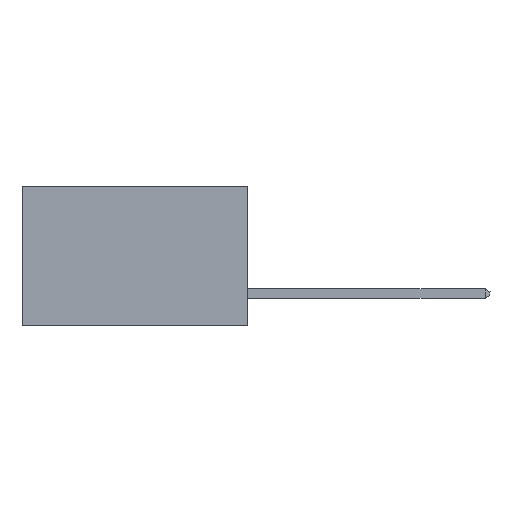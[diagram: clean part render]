
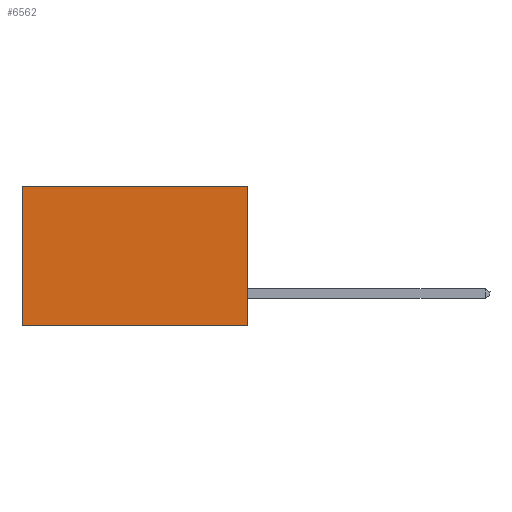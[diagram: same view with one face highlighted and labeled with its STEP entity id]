
A CAD part, left-side view. The second image highlights one B-rep face of the part: STEP entity #6562.
In plain terms, the highlighted planar face has unit normal (-1, 0, 0).
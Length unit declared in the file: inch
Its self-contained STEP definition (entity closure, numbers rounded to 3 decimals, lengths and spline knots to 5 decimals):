
#24 = VERTEX_POINT ( 'NONE', #7957 ) ;
#61 = EDGE_CURVE ( 'NONE', #7415, #7233, #4012, .T. ) ;
#595 = CARTESIAN_POINT ( 'NONE',  ( 0.2615, 0., -0.37 ) ) ;
#626 = CARTESIAN_POINT ( 'NONE',  ( 0.2615, 0., -0.37 ) ) ;
#1001 = DIRECTION ( 'NONE',  ( 1., 0., 0. ) ) ;
#1233 = LINE ( 'NONE', #626, #4310 ) ;
#1252 = DIRECTION ( 'NONE',  ( 0., 0., -1. ) ) ;
#1678 = VERTEX_POINT ( 'NONE', #8600 ) ;
#1913 = EDGE_CURVE ( 'NONE', #1678, #7233, #5636, .T. ) ;
#2053 = DIRECTION ( 'NONE',  ( 0., 0., -1. ) ) ;
#2058 = ORIENTED_EDGE ( 'NONE', *, *, #7206, .T. ) ;
#2691 = VECTOR ( 'NONE', #4969, 39.37008 ) ;
#2714 = EDGE_LOOP ( 'NONE', ( #5445, #8062, #8939, #2058 ) ) ;
#3374 = CARTESIAN_POINT ( 'NONE',  ( 0.2615, 0.6, -0.37 ) ) ;
#3808 = DIRECTION ( 'NONE',  ( 0., 0., -1. ) ) ;
#3899 = PLANE ( 'NONE',  #4866 ) ;
#4012 = LINE ( 'NONE', #3374, #8035 ) ;
#4310 = VECTOR ( 'NONE', #2053, 39.37008 ) ;
#4866 = AXIS2_PLACEMENT_3D ( 'NONE', #6674, #1001, #3808 ) ;
#4880 = CARTESIAN_POINT ( 'NONE',  ( 0.2615, 0., 0. ) ) ;
#4969 = DIRECTION ( 'NONE',  ( 0., 1., 0. ) ) ;
#5445 = ORIENTED_EDGE ( 'NONE', *, *, #61, .T. ) ;
#5636 = LINE ( 'NONE', #595, #6401 ) ;
#6177 = DIRECTION ( 'NONE',  ( 0., 1., 0. ) ) ;
#6244 = LINE ( 'NONE', #4880, #2691 ) ;
#6401 = VECTOR ( 'NONE', #6177, 39.37008 ) ;
#6562 = ADVANCED_FACE ( 'NONE', ( #7353 ), #3899, .F. ) ;
#6674 = CARTESIAN_POINT ( 'NONE',  ( 0.2615, 0., -0.37 ) ) ;
#7206 = EDGE_CURVE ( 'NONE', #24, #7415, #6244, .T. ) ;
#7233 = VERTEX_POINT ( 'NONE', #7641 ) ;
#7353 = FACE_OUTER_BOUND ( 'NONE', #2714, .T. ) ;
#7368 = CARTESIAN_POINT ( 'NONE',  ( 0.2615, 0.6, 0. ) ) ;
#7415 = VERTEX_POINT ( 'NONE', #7368 ) ;
#7641 = CARTESIAN_POINT ( 'NONE',  ( 0.2615, 0.6, -0.37 ) ) ;
#7957 = CARTESIAN_POINT ( 'NONE',  ( 0.2615, 0., 0. ) ) ;
#8007 = EDGE_CURVE ( 'NONE', #24, #1678, #1233, .T. ) ;
#8035 = VECTOR ( 'NONE', #1252, 39.37008 ) ;
#8062 = ORIENTED_EDGE ( 'NONE', *, *, #1913, .F. ) ;
#8600 = CARTESIAN_POINT ( 'NONE',  ( 0.2615, 0., -0.37 ) ) ;
#8939 = ORIENTED_EDGE ( 'NONE', *, *, #8007, .F. ) ;
